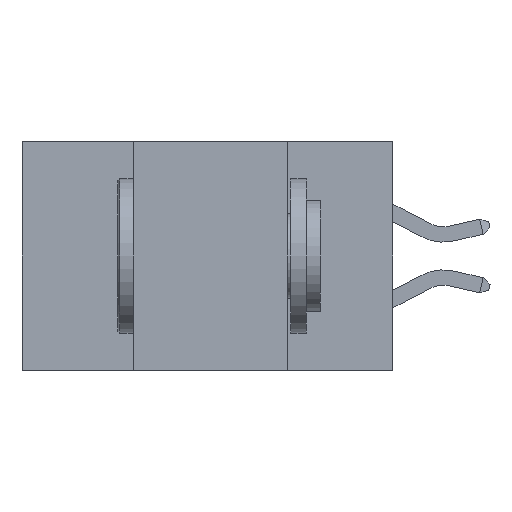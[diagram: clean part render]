
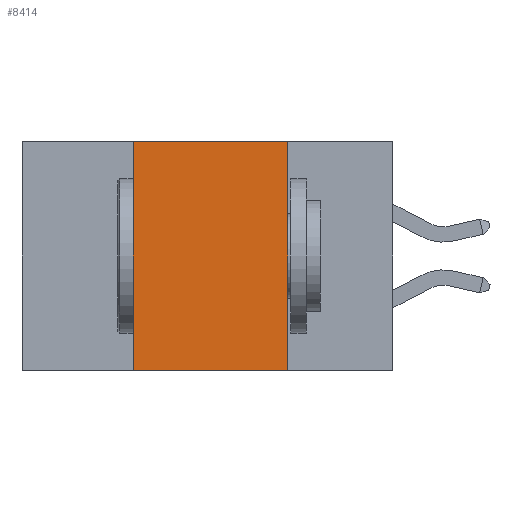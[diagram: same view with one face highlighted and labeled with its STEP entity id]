
A CAD part, left-side view. The second image highlights one B-rep face of the part: STEP entity #8414.
In plain terms, the highlighted planar face has unit normal (-1, 0, 0).
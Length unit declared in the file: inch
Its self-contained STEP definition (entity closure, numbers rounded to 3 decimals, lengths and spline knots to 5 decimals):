
#108 = CARTESIAN_POINT ( 'NONE',  ( 0., 0.17, 0. ) ) ;
#182 = VERTEX_POINT ( 'NONE', #108 ) ;
#1735 = DIRECTION ( 'NONE',  ( 0., 0., 1. ) ) ;
#2065 = DIRECTION ( 'NONE',  ( 0., 0., -1. ) ) ;
#2440 = VECTOR ( 'NONE', #4104, 39.37008 ) ;
#2455 = CARTESIAN_POINT ( 'NONE',  ( 0., 0.6, -0.37 ) ) ;
#2464 = LINE ( 'NONE', #10547, #12349 ) ;
#2909 = DIRECTION ( 'NONE',  ( 1., 0., 0. ) ) ;
#3148 = EDGE_CURVE ( 'NONE', #21497, #13674, #7146, .T. ) ;
#4104 = DIRECTION ( 'NONE',  ( 0., -1., 0. ) ) ;
#4585 = EDGE_LOOP ( 'NONE', ( #8239, #8531, #14275, #12354 ) ) ;
#5549 = LINE ( 'NONE', #12596, #18417 ) ;
#5555 = EDGE_CURVE ( 'NONE', #19874, #182, #8386, .T. ) ;
#6656 = FACE_OUTER_BOUND ( 'NONE', #4585, .T. ) ;
#7146 = LINE ( 'NONE', #2455, #2440 ) ;
#8239 = ORIENTED_EDGE ( 'NONE', *, *, #22756, .F. ) ;
#8386 = LINE ( 'NONE', #12978, #13030 ) ;
#8414 = ADVANCED_FACE ( 'NONE', ( #6656 ), #9890, .F. ) ;
#8458 = CARTESIAN_POINT ( 'NONE',  ( 0., 0.42, 0. ) ) ;
#8531 = ORIENTED_EDGE ( 'NONE', *, *, #5555, .F. ) ;
#9890 = PLANE ( 'NONE',  #21795 ) ;
#10547 = CARTESIAN_POINT ( 'NONE',  ( 0., 0.42, 0. ) ) ;
#12349 = VECTOR ( 'NONE', #1735, 39.37008 ) ;
#12354 = ORIENTED_EDGE ( 'NONE', *, *, #3148, .T. ) ;
#12596 = CARTESIAN_POINT ( 'NONE',  ( 0., 0.17, 0. ) ) ;
#12978 = CARTESIAN_POINT ( 'NONE',  ( 0., 0.6, 0. ) ) ;
#13030 = VECTOR ( 'NONE', #20039, 39.37008 ) ;
#13674 = VERTEX_POINT ( 'NONE', #18179 ) ;
#14275 = ORIENTED_EDGE ( 'NONE', *, *, #19307, .F. ) ;
#15178 = DIRECTION ( 'NONE',  ( 0., 0., -1. ) ) ;
#18179 = CARTESIAN_POINT ( 'NONE',  ( 0., 0.17, -0.37 ) ) ;
#18417 = VECTOR ( 'NONE', #2065, 39.37008 ) ;
#18628 = CARTESIAN_POINT ( 'NONE',  ( 0., 0.6, 0. ) ) ;
#19307 = EDGE_CURVE ( 'NONE', #21497, #19874, #2464, .T. ) ;
#19874 = VERTEX_POINT ( 'NONE', #8458 ) ;
#20039 = DIRECTION ( 'NONE',  ( 0., -1., 0. ) ) ;
#20974 = CARTESIAN_POINT ( 'NONE',  ( 0., 0.42, -0.37 ) ) ;
#21497 = VERTEX_POINT ( 'NONE', #20974 ) ;
#21795 = AXIS2_PLACEMENT_3D ( 'NONE', #18628, #2909, #15178 ) ;
#22756 = EDGE_CURVE ( 'NONE', #182, #13674, #5549, .T. ) ;
